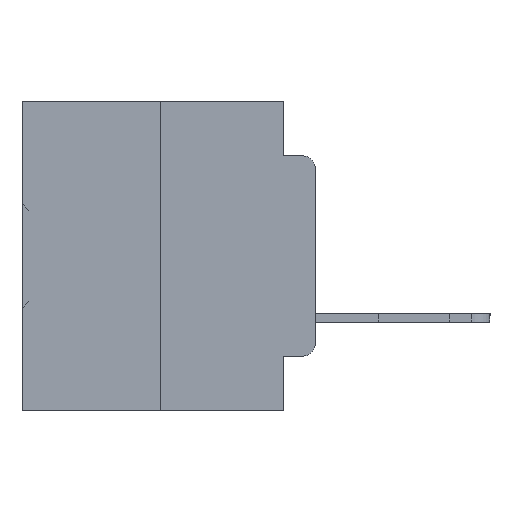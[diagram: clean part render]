
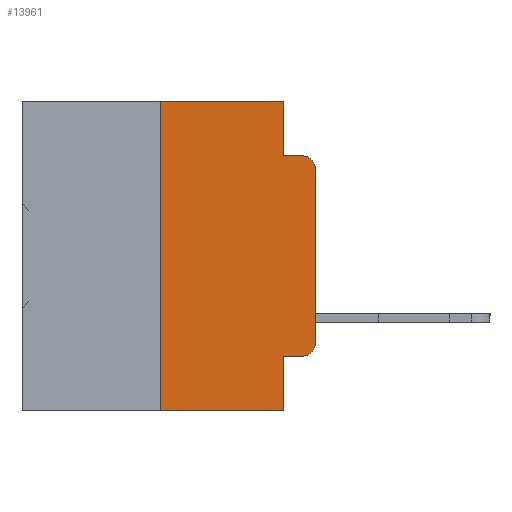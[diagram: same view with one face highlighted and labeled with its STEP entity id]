
A CAD part, left-side view. The second image highlights one B-rep face of the part: STEP entity #13961.
In plain terms, the highlighted planar face has unit normal (-1, 0, 0).
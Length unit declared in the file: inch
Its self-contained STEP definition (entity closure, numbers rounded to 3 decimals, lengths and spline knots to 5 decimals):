
#689 = VERTEX_POINT ( 'NONE', #29340 ) ;
#847 = LINE ( 'NONE', #23414, #7405 ) ;
#876 = DIRECTION ( 'NONE',  ( 0., 0., 1. ) ) ;
#1124 = DIRECTION ( 'NONE',  ( 0., -1., 0. ) ) ;
#2212 = ORIENTED_EDGE ( 'NONE', *, *, #24342, .F. ) ;
#4167 = CARTESIAN_POINT ( 'NONE',  ( 0., 0.051, 0. ) ) ;
#4304 = CARTESIAN_POINT ( 'NONE',  ( 0., 0.051, 0. ) ) ;
#5961 = LINE ( 'NONE', #4167, #27573 ) ;
#6324 = CIRCLE ( 'NONE', #19655, 0.02 ) ;
#6494 = CARTESIAN_POINT ( 'NONE',  ( 0., 0.473, 0. ) ) ;
#6512 = EDGE_LOOP ( 'NONE', ( #10545, #11850, #34343, #21159, #36104, #15398, #8768, #2212, #17170, #11413 ) ) ;
#6713 = CARTESIAN_POINT ( 'NONE',  ( 0., 0.02, -0.3915 ) ) ;
#6989 = DIRECTION ( 'NONE',  ( 0., 0., -1. ) ) ;
#7305 = EDGE_CURVE ( 'NONE', #33531, #17845, #5961, .T. ) ;
#7308 = LINE ( 'NONE', #14464, #8193 ) ;
#7405 = VECTOR ( 'NONE', #876, 39.37008 ) ;
#7836 = LINE ( 'NONE', #26340, #8715 ) ;
#8193 = VECTOR ( 'NONE', #34167, 39.37008 ) ;
#8715 = VECTOR ( 'NONE', #1124, 39.37008 ) ;
#8768 = ORIENTED_EDGE ( 'NONE', *, *, #22939, .T. ) ;
#9538 = DIRECTION ( 'NONE',  ( 0., 0., -1. ) ) ;
#9597 = CARTESIAN_POINT ( 'NONE',  ( 0., 0.02, -0.1085 ) ) ;
#10157 = VERTEX_POINT ( 'NONE', #16144 ) ;
#10545 = ORIENTED_EDGE ( 'NONE', *, *, #31872, .T. ) ;
#11054 = EDGE_CURVE ( 'NONE', #32491, #22579, #6324, .T. ) ;
#11413 = ORIENTED_EDGE ( 'NONE', *, *, #11054, .T. ) ;
#11850 = ORIENTED_EDGE ( 'NONE', *, *, #28118, .T. ) ;
#12442 = DIRECTION ( 'NONE',  ( 0., 0., -1. ) ) ;
#12973 = DIRECTION ( 'NONE',  ( 0., 0., 1. ) ) ;
#13278 = VECTOR ( 'NONE', #15510, 39.37008 ) ;
#13961 = ADVANCED_FACE ( 'NONE', ( #25762 ), #17718, .F. ) ;
#14161 = LINE ( 'NONE', #4304, #13278 ) ;
#14464 = CARTESIAN_POINT ( 'NONE',  ( 0., 0.473, 0. ) ) ;
#14874 = EDGE_CURVE ( 'NONE', #17845, #24352, #31414, .T. ) ;
#15398 = ORIENTED_EDGE ( 'NONE', *, *, #32580, .F. ) ;
#15510 = DIRECTION ( 'NONE',  ( 0., 0., -1. ) ) ;
#16028 = VECTOR ( 'NONE', #26040, 39.37008 ) ;
#16144 = CARTESIAN_POINT ( 'NONE',  ( 0., 0.051, -0.4115 ) ) ;
#16169 = CARTESIAN_POINT ( 'NONE',  ( 0., 0.051, -0.0885 ) ) ;
#17170 = ORIENTED_EDGE ( 'NONE', *, *, #26930, .T. ) ;
#17315 = VECTOR ( 'NONE', #21859, 39.37008 ) ;
#17718 = PLANE ( 'NONE',  #27734 ) ;
#17838 = DIRECTION ( 'NONE',  ( 0., 0., -1. ) ) ;
#17845 = VERTEX_POINT ( 'NONE', #32953 ) ;
#19121 = CARTESIAN_POINT ( 'NONE',  ( 0., 0.051, -0.5 ) ) ;
#19320 = CARTESIAN_POINT ( 'NONE',  ( 0., 0.25, -0.5 ) ) ;
#19655 = AXIS2_PLACEMENT_3D ( 'NONE', #6713, #26442, #9538 ) ;
#20849 = EDGE_CURVE ( 'NONE', #27639, #33531, #7308, .T. ) ;
#21159 = ORIENTED_EDGE ( 'NONE', *, *, #7305, .F. ) ;
#21528 = VERTEX_POINT ( 'NONE', #19121 ) ;
#21859 = DIRECTION ( 'NONE',  ( 0., -1., 0. ) ) ;
#22579 = VERTEX_POINT ( 'NONE', #30012 ) ;
#22939 = EDGE_CURVE ( 'NONE', #28944, #21528, #24424, .T. ) ;
#23414 = CARTESIAN_POINT ( 'NONE',  ( 0., 0.25, 0. ) ) ;
#24342 = EDGE_CURVE ( 'NONE', #10157, #21528, #14161, .T. ) ;
#24352 = VERTEX_POINT ( 'NONE', #32510 ) ;
#24424 = LINE ( 'NONE', #34411, #16028 ) ;
#25532 = LINE ( 'NONE', #32677, #31260 ) ;
#25762 = FACE_OUTER_BOUND ( 'NONE', #6512, .T. ) ;
#26040 = DIRECTION ( 'NONE',  ( 0., -1., 0. ) ) ;
#26340 = CARTESIAN_POINT ( 'NONE',  ( 0., 0.051, -0.4115 ) ) ;
#26442 = DIRECTION ( 'NONE',  ( -1., 0., 0. ) ) ;
#26930 = EDGE_CURVE ( 'NONE', #10157, #32491, #7836, .T. ) ;
#27573 = VECTOR ( 'NONE', #6989, 39.37008 ) ;
#27639 = VERTEX_POINT ( 'NONE', #32568 ) ;
#27734 = AXIS2_PLACEMENT_3D ( 'NONE', #6494, #34710, #17838 ) ;
#28118 = EDGE_CURVE ( 'NONE', #689, #24352, #31113, .T. ) ;
#28692 = CARTESIAN_POINT ( 'NONE',  ( 0., 0.02, -0.4115 ) ) ;
#28944 = VERTEX_POINT ( 'NONE', #19320 ) ;
#29340 = CARTESIAN_POINT ( 'NONE',  ( 0., 0., -0.1085 ) ) ;
#29341 = DIRECTION ( 'NONE',  ( -1., 0., 0. ) ) ;
#29951 = AXIS2_PLACEMENT_3D ( 'NONE', #9597, #29341, #12442 ) ;
#30012 = CARTESIAN_POINT ( 'NONE',  ( 0., 0., -0.3915 ) ) ;
#31113 = CIRCLE ( 'NONE', #29951, 0.02 ) ;
#31260 = VECTOR ( 'NONE', #12973, 39.37008 ) ;
#31414 = LINE ( 'NONE', #16169, #17315 ) ;
#31872 = EDGE_CURVE ( 'NONE', #22579, #689, #25532, .T. ) ;
#32491 = VERTEX_POINT ( 'NONE', #28692 ) ;
#32510 = CARTESIAN_POINT ( 'NONE',  ( 0., 0.02, -0.0885 ) ) ;
#32568 = CARTESIAN_POINT ( 'NONE',  ( 0., 0.25, 0. ) ) ;
#32580 = EDGE_CURVE ( 'NONE', #28944, #27639, #847, .T. ) ;
#32677 = CARTESIAN_POINT ( 'NONE',  ( 0., 0., 0. ) ) ;
#32953 = CARTESIAN_POINT ( 'NONE',  ( 0., 0.051, -0.0885 ) ) ;
#33516 = CARTESIAN_POINT ( 'NONE',  ( 0., 0.051, 0. ) ) ;
#33531 = VERTEX_POINT ( 'NONE', #33516 ) ;
#34167 = DIRECTION ( 'NONE',  ( 0., -1., 0. ) ) ;
#34343 = ORIENTED_EDGE ( 'NONE', *, *, #14874, .F. ) ;
#34411 = CARTESIAN_POINT ( 'NONE',  ( 0., 0.473, -0.5 ) ) ;
#34710 = DIRECTION ( 'NONE',  ( 1., 0., 0. ) ) ;
#36104 = ORIENTED_EDGE ( 'NONE', *, *, #20849, .F. ) ;
